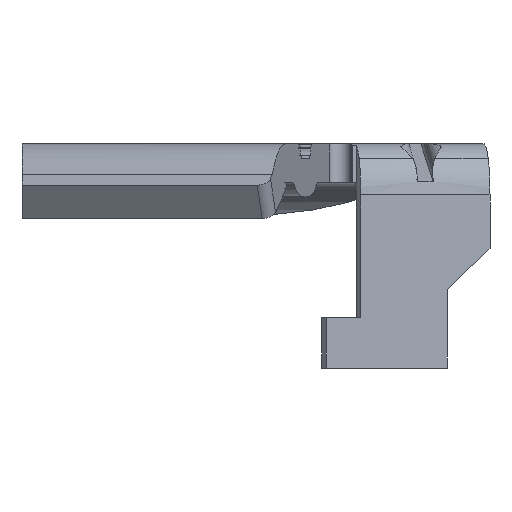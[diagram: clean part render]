
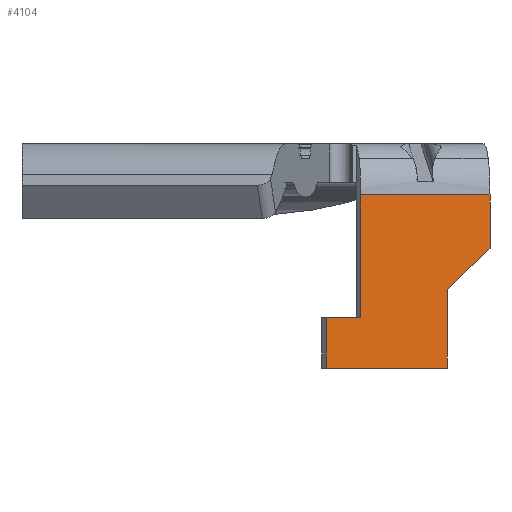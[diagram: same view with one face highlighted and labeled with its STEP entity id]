
A CAD part, left-side view. The second image highlights one B-rep face of the part: STEP entity #4104.
In plain terms, the highlighted planar face has unit normal (-0.993, -0.117, 0).
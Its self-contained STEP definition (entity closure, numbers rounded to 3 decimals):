
#227 = CARTESIAN_POINT ( 'NONE',  ( -62.313, -8.285, 0. ) ) ;
#234 = VECTOR ( 'NONE', #1790, 1000. ) ;
#242 = EDGE_CURVE ( 'NONE', #3611, #2398, #2843, .T. ) ;
#310 = EDGE_CURVE ( 'NONE', #1972, #3611, #3947, .T. ) ;
#421 = VERTEX_POINT ( 'NONE', #2812 ) ;
#438 = CARTESIAN_POINT ( 'NONE',  ( -62.313, -8.285, -6.153 ) ) ;
#442 = EDGE_CURVE ( 'NONE', #1506, #2398, #3977, .T. ) ;
#486 = CARTESIAN_POINT ( 'NONE',  ( -61.706, -13.425, -1.264 ) ) ;
#500 = ORIENTED_EDGE ( 'NONE', *, *, #989, .T. ) ;
#910 = ORIENTED_EDGE ( 'NONE', *, *, #442, .F. ) ;
#922 = CARTESIAN_POINT ( 'NONE',  ( -61.706, -13.425, -8.16 ) ) ;
#934 = PLANE ( 'NONE',  #3448 ) ;
#942 = LINE ( 'NONE', #1437, #1942 ) ;
#989 = EDGE_CURVE ( 'NONE', #1303, #421, #942, .T. ) ;
#1020 = CARTESIAN_POINT ( 'NONE',  ( -62.313, -8.285, -1.264 ) ) ;
#1068 = LINE ( 'NONE', #438, #2703 ) ;
#1087 = CARTESIAN_POINT ( 'NONE',  ( -62.477, -6.898, -8.16 ) ) ;
#1110 = LINE ( 'NONE', #922, #2732 ) ;
#1240 = VERTEX_POINT ( 'NONE', #1087 ) ;
#1245 = ORIENTED_EDGE ( 'NONE', *, *, #3397, .T. ) ;
#1248 = DIRECTION ( 'NONE',  ( 0.117, -0.993, 0. ) ) ;
#1272 = CARTESIAN_POINT ( 'NONE',  ( -62.279, -8.577, -1.264 ) ) ;
#1287 = DIRECTION ( 'NONE',  ( -0.993, -0.117, 0. ) ) ;
#1303 = VERTEX_POINT ( 'NONE', #1020 ) ;
#1334 = ORIENTED_EDGE ( 'NONE', *, *, #3573, .F. ) ;
#1437 = CARTESIAN_POINT ( 'NONE',  ( -62.313, -8.285, 0. ) ) ;
#1506 = VERTEX_POINT ( 'NONE', #486 ) ;
#1570 = DIRECTION ( 'NONE',  ( 0., 0., -1. ) ) ;
#1790 = DIRECTION ( 'NONE',  ( 0., 0., 1. ) ) ;
#1942 = VECTOR ( 'NONE', #1570, 1000. ) ;
#1972 = VERTEX_POINT ( 'NONE', #2366 ) ;
#2049 = FACE_OUTER_BOUND ( 'NONE', #3669, .T. ) ;
#2163 = LINE ( 'NONE', #3645, #234 ) ;
#2366 = CARTESIAN_POINT ( 'NONE',  ( -61.907, -11.721, -8.16 ) ) ;
#2398 = VERTEX_POINT ( 'NONE', #3277 ) ;
#2420 = VECTOR ( 'NONE', #2763, 1000. ) ;
#2482 = DIRECTION ( 'NONE',  ( -0.117, 0.993, 0. ) ) ;
#2585 = ORIENTED_EDGE ( 'NONE', *, *, #2687, .F. ) ;
#2680 = CARTESIAN_POINT ( 'NONE',  ( -61.706, -13.425, 0. ) ) ;
#2687 = EDGE_CURVE ( 'NONE', #1303, #1506, #2778, .T. ) ;
#2703 = VECTOR ( 'NONE', #2482, 1000. ) ;
#2732 = VECTOR ( 'NONE', #3180, 1000. ) ;
#2763 = DIRECTION ( 'NONE',  ( 0., 0., -1. ) ) ;
#2778 = LINE ( 'NONE', #1272, #3388 ) ;
#2812 = CARTESIAN_POINT ( 'NONE',  ( -62.313, -8.285, -6.153 ) ) ;
#2843 = LINE ( 'NONE', #3433, #3547 ) ;
#3180 = DIRECTION ( 'NONE',  ( -0.117, 0.993, 0. ) ) ;
#3183 = DIRECTION ( 'NONE',  ( 0., 0., 1. ) ) ;
#3191 = CARTESIAN_POINT ( 'NONE',  ( -61.907, -11.721, -4.08 ) ) ;
#3277 = CARTESIAN_POINT ( 'NONE',  ( -61.706, -13.425, -3.4 ) ) ;
#3332 = EDGE_CURVE ( 'NONE', #1240, #3513, #2163, .T. ) ;
#3339 = ORIENTED_EDGE ( 'NONE', *, *, #3332, .F. ) ;
#3373 = ORIENTED_EDGE ( 'NONE', *, *, #242, .T. ) ;
#3388 = VECTOR ( 'NONE', #1248, 1000. ) ;
#3397 = EDGE_CURVE ( 'NONE', #421, #3513, #1068, .T. ) ;
#3418 = CARTESIAN_POINT ( 'NONE',  ( -62.477, -6.898, -6.153 ) ) ;
#3433 = CARTESIAN_POINT ( 'NONE',  ( -61.868, -12.055, -4.701 ) ) ;
#3443 = DIRECTION ( 'NONE',  ( 0.085, -0.723, 0.686 ) ) ;
#3448 = AXIS2_PLACEMENT_3D ( 'NONE', #227, #1287, #3490 ) ;
#3472 = CARTESIAN_POINT ( 'NONE',  ( -61.907, -11.721, -5.019 ) ) ;
#3490 = DIRECTION ( 'NONE',  ( 0.117, -0.993, 0. ) ) ;
#3513 = VERTEX_POINT ( 'NONE', #3418 ) ;
#3547 = VECTOR ( 'NONE', #3443, 1000. ) ;
#3573 = EDGE_CURVE ( 'NONE', #1972, #1240, #1110, .T. ) ;
#3611 = VERTEX_POINT ( 'NONE', #3472 ) ;
#3645 = CARTESIAN_POINT ( 'NONE',  ( -62.477, -6.898, -8.16 ) ) ;
#3669 = EDGE_LOOP ( 'NONE', ( #3373, #910, #2585, #500, #1245, #3339, #1334, #4022 ) ) ;
#3947 = LINE ( 'NONE', #3191, #3948 ) ;
#3948 = VECTOR ( 'NONE', #3183, 1000. ) ;
#3977 = LINE ( 'NONE', #2680, #2420 ) ;
#4022 = ORIENTED_EDGE ( 'NONE', *, *, #310, .T. ) ;
#4104 = ADVANCED_FACE ( 'NONE', ( #2049 ), #934, .T. ) ;
